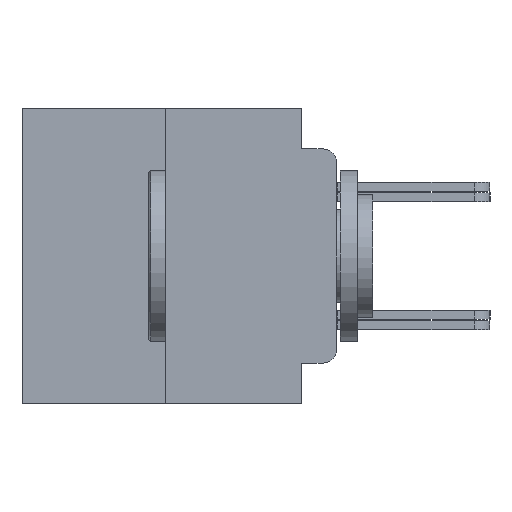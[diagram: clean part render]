
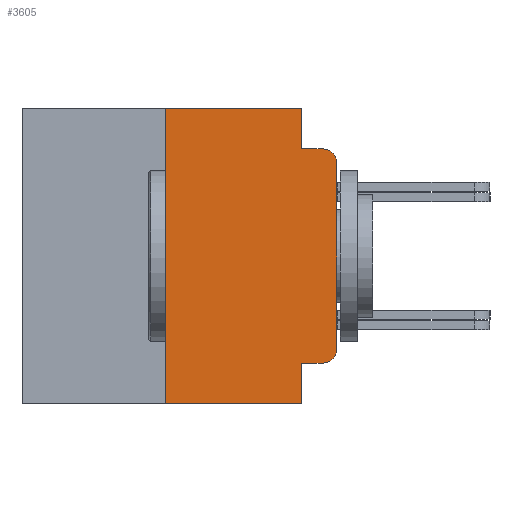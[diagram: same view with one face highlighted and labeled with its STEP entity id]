
A CAD part, left-side view. The second image highlights one B-rep face of the part: STEP entity #3605.
In plain terms, the highlighted planar face has unit normal (-1, 0, 0).
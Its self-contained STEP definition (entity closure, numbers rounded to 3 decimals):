
#55 = DIRECTION ( 'NONE',  ( 0., -1., 0. ) ) ;
#472 = VERTEX_POINT ( 'NONE', #10744 ) ;
#1502 = EDGE_CURVE ( 'NONE', #6981, #13111, #28340, .T. ) ;
#2451 = CARTESIAN_POINT ( 'NONE',  ( -75.603, 11.684, 5.486 ) ) ;
#2653 = ORIENTED_EDGE ( 'NONE', *, *, #9767, .T. ) ;
#2674 = VECTOR ( 'NONE', #28026, 1000. ) ;
#3299 = ORIENTED_EDGE ( 'NONE', *, *, #16318, .F. ) ;
#3503 = VECTOR ( 'NONE', #18306, 1000. ) ;
#3605 = ADVANCED_FACE ( 'NONE', ( #12131 ), #18052, .F. ) ;
#5010 = VERTEX_POINT ( 'NONE', #15965 ) ;
#5228 = EDGE_LOOP ( 'NONE', ( #15178, #16792, #10439, #13957, #7284, #15580, #10784, #22785, #2653, #3299 ) ) ;
#5283 = LINE ( 'NONE', #14005, #3503 ) ;
#5911 = CARTESIAN_POINT ( 'NONE',  ( -75.603, 1.295, -3.975 ) ) ;
#6346 = CIRCLE ( 'NONE', #15725, 0.508 ) ;
#6981 = VERTEX_POINT ( 'NONE', #20177 ) ;
#7250 = EDGE_CURVE ( 'NONE', #9092, #22314, #24874, .T. ) ;
#7284 = ORIENTED_EDGE ( 'NONE', *, *, #1502, .F. ) ;
#7554 = CARTESIAN_POINT ( 'NONE',  ( -75.603, 0., -3.467 ) ) ;
#9092 = VERTEX_POINT ( 'NONE', #7554 ) ;
#9767 = EDGE_CURVE ( 'NONE', #10775, #5010, #17813, .T. ) ;
#10112 = EDGE_CURVE ( 'NONE', #10775, #23470, #5283, .T. ) ;
#10402 = DIRECTION ( 'NONE',  ( 0., -1., 0. ) ) ;
#10439 = ORIENTED_EDGE ( 'NONE', *, *, #7250, .T. ) ;
#10744 = CARTESIAN_POINT ( 'NONE',  ( -75.603, 1.295, 5.486 ) ) ;
#10775 = VERTEX_POINT ( 'NONE', #15961 ) ;
#10784 = ORIENTED_EDGE ( 'NONE', *, *, #16658, .F. ) ;
#11405 = VECTOR ( 'NONE', #10402, 1000. ) ;
#12131 = FACE_OUTER_BOUND ( 'NONE', #5228, .T. ) ;
#12167 = DIRECTION ( 'NONE',  ( -1., 0., 0. ) ) ;
#12257 = CARTESIAN_POINT ( 'NONE',  ( -75.603, 1.295, 3.975 ) ) ;
#12304 = VECTOR ( 'NONE', #23671, 1000. ) ;
#12536 = CIRCLE ( 'NONE', #25144, 0.508 ) ;
#13111 = VERTEX_POINT ( 'NONE', #29371 ) ;
#13159 = DIRECTION ( 'NONE',  ( 0., 0., -1. ) ) ;
#13365 = DIRECTION ( 'NONE',  ( 1., 0., 0. ) ) ;
#13764 = CARTESIAN_POINT ( 'NONE',  ( -75.603, 0., 3.467 ) ) ;
#13957 = ORIENTED_EDGE ( 'NONE', *, *, #19714, .T. ) ;
#14005 = CARTESIAN_POINT ( 'NONE',  ( -75.603, 6.35, -5.486 ) ) ;
#15033 = CARTESIAN_POINT ( 'NONE',  ( -75.603, 0.508, -3.975 ) ) ;
#15178 = ORIENTED_EDGE ( 'NONE', *, *, #18370, .T. ) ;
#15559 = CARTESIAN_POINT ( 'NONE',  ( -75.603, 1.295, -3.975 ) ) ;
#15580 = ORIENTED_EDGE ( 'NONE', *, *, #23011, .F. ) ;
#15725 = AXIS2_PLACEMENT_3D ( 'NONE', #22240, #22436, #27151 ) ;
#15949 = DIRECTION ( 'NONE',  ( 0., 0., -1. ) ) ;
#15961 = CARTESIAN_POINT ( 'NONE',  ( -75.603, 6.35, -5.486 ) ) ;
#15965 = CARTESIAN_POINT ( 'NONE',  ( -75.603, 1.295, -5.486 ) ) ;
#16318 = EDGE_CURVE ( 'NONE', #19725, #5010, #16946, .T. ) ;
#16522 = CARTESIAN_POINT ( 'NONE',  ( -75.603, 1.295, 0. ) ) ;
#16658 = EDGE_CURVE ( 'NONE', #23470, #472, #22319, .T. ) ;
#16792 = ORIENTED_EDGE ( 'NONE', *, *, #18117, .T. ) ;
#16946 = LINE ( 'NONE', #28578, #17661 ) ;
#17279 = CARTESIAN_POINT ( 'NONE',  ( -75.603, 11.684, -5.486 ) ) ;
#17661 = VECTOR ( 'NONE', #13159, 1000. ) ;
#17813 = LINE ( 'NONE', #17279, #11405 ) ;
#18052 = PLANE ( 'NONE',  #20037 ) ;
#18117 = EDGE_CURVE ( 'NONE', #25915, #9092, #12536, .T. ) ;
#18306 = DIRECTION ( 'NONE',  ( 0., 0., 1. ) ) ;
#18370 = EDGE_CURVE ( 'NONE', #19725, #25915, #22210, .T. ) ;
#19068 = DIRECTION ( 'NONE',  ( 0., 0., -1. ) ) ;
#19170 = CARTESIAN_POINT ( 'NONE',  ( -75.603, 0.508, -3.467 ) ) ;
#19714 = EDGE_CURVE ( 'NONE', #22314, #13111, #6346, .T. ) ;
#19725 = VERTEX_POINT ( 'NONE', #5911 ) ;
#20037 = AXIS2_PLACEMENT_3D ( 'NONE', #25110, #13365, #15949 ) ;
#20123 = CARTESIAN_POINT ( 'NONE',  ( -75.603, 6.35, 5.486 ) ) ;
#20177 = CARTESIAN_POINT ( 'NONE',  ( -75.603, 1.295, 3.975 ) ) ;
#22210 = LINE ( 'NONE', #15559, #25808 ) ;
#22240 = CARTESIAN_POINT ( 'NONE',  ( -75.603, 0.508, 3.467 ) ) ;
#22314 = VERTEX_POINT ( 'NONE', #13764 ) ;
#22319 = LINE ( 'NONE', #2451, #24476 ) ;
#22436 = DIRECTION ( 'NONE',  ( -1., 0., 0. ) ) ;
#22785 = ORIENTED_EDGE ( 'NONE', *, *, #10112, .F. ) ;
#23011 = EDGE_CURVE ( 'NONE', #472, #6981, #25288, .T. ) ;
#23470 = VERTEX_POINT ( 'NONE', #20123 ) ;
#23671 = DIRECTION ( 'NONE',  ( 0., 0., 1. ) ) ;
#24476 = VECTOR ( 'NONE', #55, 1000. ) ;
#24805 = DIRECTION ( 'NONE',  ( 0., -1., 0. ) ) ;
#24874 = LINE ( 'NONE', #27949, #12304 ) ;
#25110 = CARTESIAN_POINT ( 'NONE',  ( -75.603, 11.684, 5.486 ) ) ;
#25144 = AXIS2_PLACEMENT_3D ( 'NONE', #19170, #12167, #19068 ) ;
#25288 = LINE ( 'NONE', #16522, #2674 ) ;
#25808 = VECTOR ( 'NONE', #24805, 1000. ) ;
#25915 = VERTEX_POINT ( 'NONE', #15033 ) ;
#26109 = DIRECTION ( 'NONE',  ( 0., -1., 0. ) ) ;
#27151 = DIRECTION ( 'NONE',  ( 0., 0., -1. ) ) ;
#27949 = CARTESIAN_POINT ( 'NONE',  ( -75.603, 0., 5.486 ) ) ;
#28026 = DIRECTION ( 'NONE',  ( 0., 0., -1. ) ) ;
#28340 = LINE ( 'NONE', #12257, #28719 ) ;
#28578 = CARTESIAN_POINT ( 'NONE',  ( -75.603, 1.295, 0. ) ) ;
#28719 = VECTOR ( 'NONE', #26109, 1000. ) ;
#29371 = CARTESIAN_POINT ( 'NONE',  ( -75.603, 0.508, 3.975 ) ) ;
